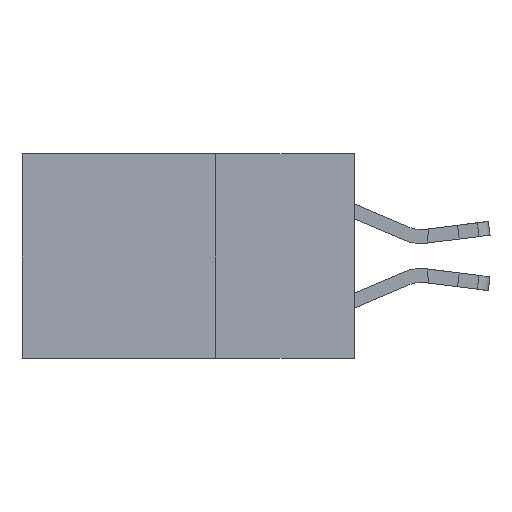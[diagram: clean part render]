
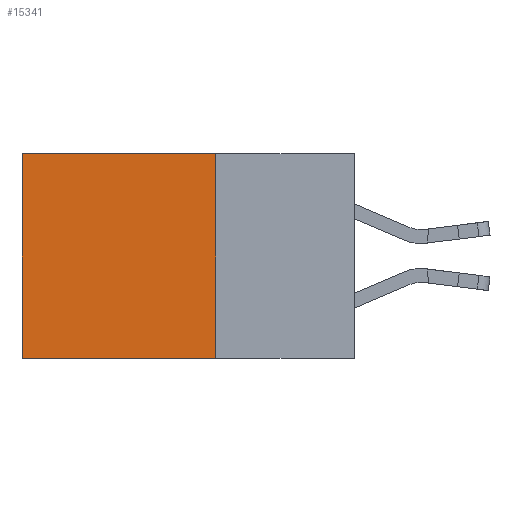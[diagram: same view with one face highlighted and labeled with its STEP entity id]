
A CAD part, left-side view. The second image highlights one B-rep face of the part: STEP entity #15341.
In plain terms, the highlighted planar face has unit normal (-1, 0, 0).
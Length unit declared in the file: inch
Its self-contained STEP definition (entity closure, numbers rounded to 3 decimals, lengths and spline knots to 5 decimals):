
#1169 = AXIS2_PLACEMENT_3D ( 'NONE', #6226, #10253, #14849 ) ;
#1636 = VECTOR ( 'NONE', #3063, 39.37008 ) ;
#2244 = EDGE_LOOP ( 'NONE', ( #13786, #15382, #4047, #3893 ) ) ;
#2373 = DIRECTION ( 'NONE',  ( 0., 0., -1. ) ) ;
#2503 = VECTOR ( 'NONE', #7564, 39.37008 ) ;
#2851 = VERTEX_POINT ( 'NONE', #5274 ) ;
#3040 = VECTOR ( 'NONE', #5684, 39.37008 ) ;
#3063 = DIRECTION ( 'NONE',  ( 0., 1., 0. ) ) ;
#3893 = ORIENTED_EDGE ( 'NONE', *, *, #9845, .T. ) ;
#4000 = VERTEX_POINT ( 'NONE', #6022 ) ;
#4047 = ORIENTED_EDGE ( 'NONE', *, *, #5132, .F. ) ;
#4715 = VECTOR ( 'NONE', #2373, 39.37008 ) ;
#5035 = LINE ( 'NONE', #14941, #4715 ) ;
#5132 = EDGE_CURVE ( 'NONE', #2851, #11161, #5600, .T. ) ;
#5274 = CARTESIAN_POINT ( 'NONE',  ( 0.2615, 0.25, 0. ) ) ;
#5600 = LINE ( 'NONE', #12821, #3040 ) ;
#5684 = DIRECTION ( 'NONE',  ( 0., 0., -1. ) ) ;
#6022 = CARTESIAN_POINT ( 'NONE',  ( 0.2615, 0.6, 0. ) ) ;
#6226 = CARTESIAN_POINT ( 'NONE',  ( 0.2615, 0.25, -0.37 ) ) ;
#6432 = CARTESIAN_POINT ( 'NONE',  ( 0.2615, 0.6, -0.37 ) ) ;
#7564 = DIRECTION ( 'NONE',  ( 0., 1., 0. ) ) ;
#7785 = PLANE ( 'NONE',  #1169 ) ;
#9250 = FACE_OUTER_BOUND ( 'NONE', #2244, .T. ) ;
#9318 = LINE ( 'NONE', #17390, #2503 ) ;
#9492 = EDGE_CURVE ( 'NONE', #11161, #16277, #9318, .T. ) ;
#9845 = EDGE_CURVE ( 'NONE', #2851, #4000, #15643, .T. ) ;
#10253 = DIRECTION ( 'NONE',  ( 1., 0., 0. ) ) ;
#11161 = VERTEX_POINT ( 'NONE', #15471 ) ;
#12821 = CARTESIAN_POINT ( 'NONE',  ( 0.2615, 0.25, -0.37 ) ) ;
#13786 = ORIENTED_EDGE ( 'NONE', *, *, #16671, .T. ) ;
#14325 = CARTESIAN_POINT ( 'NONE',  ( 0.2615, 0.25, 0. ) ) ;
#14849 = DIRECTION ( 'NONE',  ( 0., 0., -1. ) ) ;
#14941 = CARTESIAN_POINT ( 'NONE',  ( 0.2615, 0.6, -0.37 ) ) ;
#15341 = ADVANCED_FACE ( 'NONE', ( #9250 ), #7785, .F. ) ;
#15382 = ORIENTED_EDGE ( 'NONE', *, *, #9492, .F. ) ;
#15471 = CARTESIAN_POINT ( 'NONE',  ( 0.2615, 0.25, -0.37 ) ) ;
#15643 = LINE ( 'NONE', #14325, #1636 ) ;
#16277 = VERTEX_POINT ( 'NONE', #6432 ) ;
#16671 = EDGE_CURVE ( 'NONE', #4000, #16277, #5035, .T. ) ;
#17390 = CARTESIAN_POINT ( 'NONE',  ( 0.2615, 0.25, -0.37 ) ) ;
